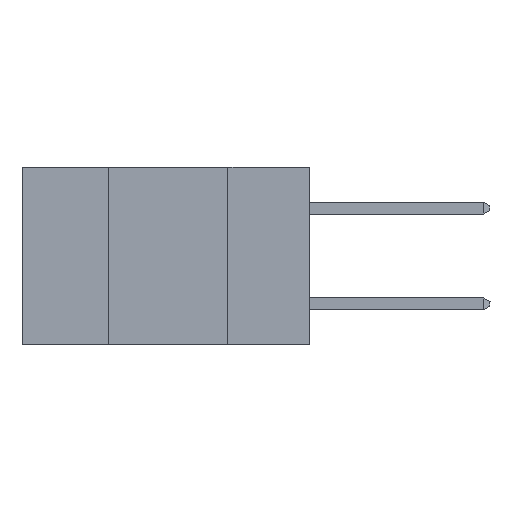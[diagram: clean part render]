
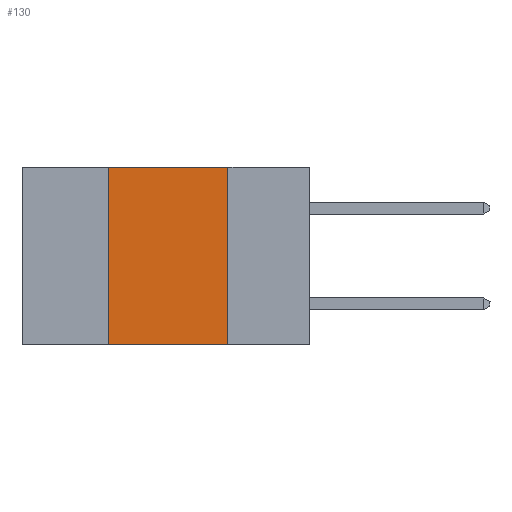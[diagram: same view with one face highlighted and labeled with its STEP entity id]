
A CAD part, left-side view. The second image highlights one B-rep face of the part: STEP entity #130.
In plain terms, the highlighted planar face has unit normal (-1, 0, 0).
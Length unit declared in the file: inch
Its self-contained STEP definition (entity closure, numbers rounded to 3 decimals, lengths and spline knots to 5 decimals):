
#3 = EDGE_CURVE ( 'NONE', #1074, #23905, #34566, .T. ) ;
#130 = ADVANCED_FACE ( 'NONE', ( #31751 ), #3656, .F. ) ;
#137 = DIRECTION ( 'NONE',  ( 0., -1., 0. ) ) ;
#1074 = VERTEX_POINT ( 'NONE', #39463 ) ;
#3461 = DIRECTION ( 'NONE',  ( 0., -1., 0. ) ) ;
#3656 = PLANE ( 'NONE',  #4248 ) ;
#4248 = AXIS2_PLACEMENT_3D ( 'NONE', #6927, #35932, #17800 ) ;
#4475 = CARTESIAN_POINT ( 'NONE',  ( 0., 0.17, 0. ) ) ;
#5209 = ORIENTED_EDGE ( 'NONE', *, *, #36412, .F. ) ;
#5446 = ORIENTED_EDGE ( 'NONE', *, *, #27888, .T. ) ;
#6853 = ORIENTED_EDGE ( 'NONE', *, *, #10438, .F. ) ;
#6927 = CARTESIAN_POINT ( 'NONE',  ( 0., 0.6, 0. ) ) ;
#7856 = EDGE_LOOP ( 'NONE', ( #5209, #6853, #8873, #5446 ) ) ;
#8873 = ORIENTED_EDGE ( 'NONE', *, *, #3, .F. ) ;
#10438 = EDGE_CURVE ( 'NONE', #23905, #27019, #13668, .T. ) ;
#10943 = DIRECTION ( 'NONE',  ( 0., 0., -1. ) ) ;
#13408 = CARTESIAN_POINT ( 'NONE',  ( 0., 0.42, 0. ) ) ;
#13668 = LINE ( 'NONE', #21074, #17752 ) ;
#14409 = CARTESIAN_POINT ( 'NONE',  ( 0., 0.17, 0. ) ) ;
#14492 = CARTESIAN_POINT ( 'NONE',  ( 0., 0.42, 0. ) ) ;
#14675 = VERTEX_POINT ( 'NONE', #33040 ) ;
#16215 = DIRECTION ( 'NONE',  ( 0., 0., 1. ) ) ;
#17752 = VECTOR ( 'NONE', #3461, 39.37008 ) ;
#17800 = DIRECTION ( 'NONE',  ( 0., 0., -1. ) ) ;
#21074 = CARTESIAN_POINT ( 'NONE',  ( 0., 0.6, 0. ) ) ;
#21255 = VECTOR ( 'NONE', #16215, 39.37008 ) ;
#21368 = LINE ( 'NONE', #14409, #35526 ) ;
#23905 = VERTEX_POINT ( 'NONE', #14492 ) ;
#23948 = VECTOR ( 'NONE', #137, 39.37008 ) ;
#27019 = VERTEX_POINT ( 'NONE', #4475 ) ;
#27888 = EDGE_CURVE ( 'NONE', #1074, #14675, #32059, .T. ) ;
#31751 = FACE_OUTER_BOUND ( 'NONE', #7856, .T. ) ;
#32059 = LINE ( 'NONE', #34995, #23948 ) ;
#33040 = CARTESIAN_POINT ( 'NONE',  ( 0., 0.17, -0.37 ) ) ;
#34566 = LINE ( 'NONE', #13408, #21255 ) ;
#34995 = CARTESIAN_POINT ( 'NONE',  ( 0., 0.6, -0.37 ) ) ;
#35526 = VECTOR ( 'NONE', #10943, 39.37008 ) ;
#35932 = DIRECTION ( 'NONE',  ( 1., 0., 0. ) ) ;
#36412 = EDGE_CURVE ( 'NONE', #27019, #14675, #21368, .T. ) ;
#39463 = CARTESIAN_POINT ( 'NONE',  ( 0., 0.42, -0.37 ) ) ;
